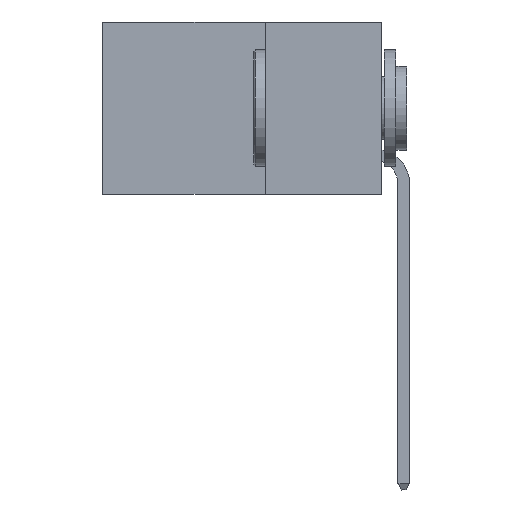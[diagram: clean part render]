
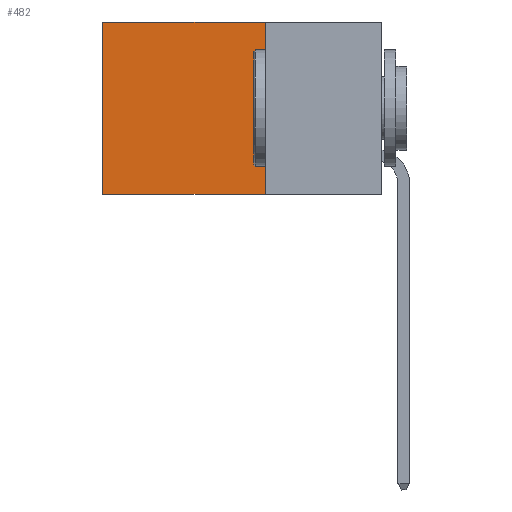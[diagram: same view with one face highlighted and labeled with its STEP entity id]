
A CAD part, left-side view. The second image highlights one B-rep face of the part: STEP entity #482.
In plain terms, the highlighted planar face has unit normal (-1, 0, 0).
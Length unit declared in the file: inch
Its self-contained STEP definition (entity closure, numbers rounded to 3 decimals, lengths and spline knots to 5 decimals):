
#482 = ADVANCED_FACE ( 'NONE', ( #6048 ), #808, .F. ) ;
#808 = PLANE ( 'NONE',  #4910 ) ;
#942 = CARTESIAN_POINT ( 'NONE',  ( 0.2875, 0.25, 0. ) ) ;
#2370 = LINE ( 'NONE', #18342, #22039 ) ;
#3813 = DIRECTION ( 'NONE',  ( 0., 0., -1. ) ) ;
#4022 = LINE ( 'NONE', #13673, #24251 ) ;
#4613 = DIRECTION ( 'NONE',  ( 0., 0., -1. ) ) ;
#4910 = AXIS2_PLACEMENT_3D ( 'NONE', #942, #9065, #9062 ) ;
#5784 = DIRECTION ( 'NONE',  ( 0., 1., 0. ) ) ;
#6048 = FACE_OUTER_BOUND ( 'NONE', #18705, .T. ) ;
#6256 = CARTESIAN_POINT ( 'NONE',  ( 0.2875, 0.6, 0. ) ) ;
#6546 = VERTEX_POINT ( 'NONE', #19785 ) ;
#6581 = CARTESIAN_POINT ( 'NONE',  ( 0.2875, 0.25, 0. ) ) ;
#6861 = VERTEX_POINT ( 'NONE', #12891 ) ;
#9062 = DIRECTION ( 'NONE',  ( 0., 0., -1. ) ) ;
#9065 = DIRECTION ( 'NONE',  ( 1., 0., 0. ) ) ;
#9455 = ORIENTED_EDGE ( 'NONE', *, *, #22126, .T. ) ;
#11106 = ORIENTED_EDGE ( 'NONE', *, *, #19476, .T. ) ;
#12064 = VERTEX_POINT ( 'NONE', #6256 ) ;
#12519 = LINE ( 'NONE', #6581, #17059 ) ;
#12891 = CARTESIAN_POINT ( 'NONE',  ( 0.2875, 0.25, 0. ) ) ;
#13613 = CARTESIAN_POINT ( 'NONE',  ( 0.2875, 0.25, -0.37 ) ) ;
#13673 = CARTESIAN_POINT ( 'NONE',  ( 0.2875, 0.25, 0. ) ) ;
#14354 = VERTEX_POINT ( 'NONE', #22323 ) ;
#14413 = DIRECTION ( 'NONE',  ( 0., 1., 0. ) ) ;
#14509 = ORIENTED_EDGE ( 'NONE', *, *, #14601, .F. ) ;
#14601 = EDGE_CURVE ( 'NONE', #6861, #14354, #4022, .T. ) ;
#15749 = EDGE_CURVE ( 'NONE', #14354, #6546, #19342, .T. ) ;
#17059 = VECTOR ( 'NONE', #14413, 39.37008 ) ;
#18342 = CARTESIAN_POINT ( 'NONE',  ( 0.2875, 0.6, 0. ) ) ;
#18705 = EDGE_LOOP ( 'NONE', ( #11106, #21961, #14509, #9455 ) ) ;
#19342 = LINE ( 'NONE', #13613, #23917 ) ;
#19476 = EDGE_CURVE ( 'NONE', #12064, #6546, #2370, .T. ) ;
#19785 = CARTESIAN_POINT ( 'NONE',  ( 0.2875, 0.6, -0.37 ) ) ;
#21961 = ORIENTED_EDGE ( 'NONE', *, *, #15749, .F. ) ;
#22039 = VECTOR ( 'NONE', #4613, 39.37008 ) ;
#22126 = EDGE_CURVE ( 'NONE', #6861, #12064, #12519, .T. ) ;
#22323 = CARTESIAN_POINT ( 'NONE',  ( 0.2875, 0.25, -0.37 ) ) ;
#23917 = VECTOR ( 'NONE', #5784, 39.37008 ) ;
#24251 = VECTOR ( 'NONE', #3813, 39.37008 ) ;
